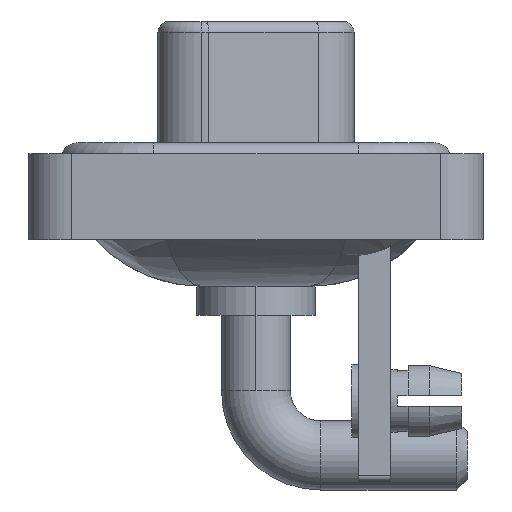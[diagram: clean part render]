
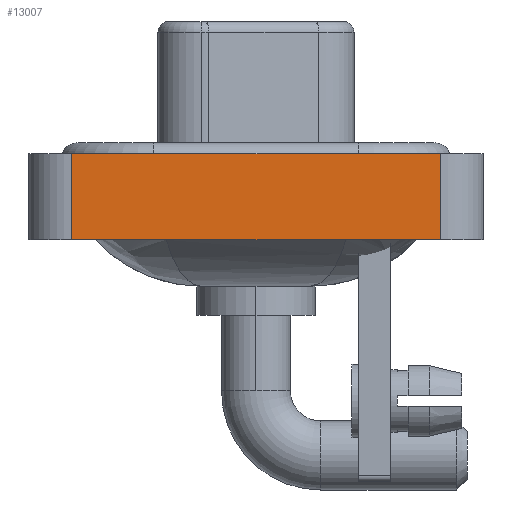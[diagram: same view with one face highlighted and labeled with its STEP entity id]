
A CAD part, left-side view. The second image highlights one B-rep face of the part: STEP entity #13007.
In plain terms, the highlighted planar face has unit normal (-1, 0, 0).
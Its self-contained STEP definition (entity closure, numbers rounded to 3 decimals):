
#25 = CARTESIAN_POINT ( 'NONE',  ( -7.35, -8.55, -3.6 ) ) ;
#1005 = AXIS2_PLACEMENT_3D ( 'NONE', #25, #5117, #6363 ) ;
#1102 = VERTEX_POINT ( 'NONE', #7436 ) ;
#1129 = CARTESIAN_POINT ( 'NONE',  ( -7.35, -8.55, -3.6 ) ) ;
#1330 = DIRECTION ( 'NONE',  ( 0., -1., 0. ) ) ;
#1501 = CARTESIAN_POINT ( 'NONE',  ( -7.35, -8.55, -3.6 ) ) ;
#2076 = VERTEX_POINT ( 'NONE', #9223 ) ;
#2586 = LINE ( 'NONE', #7348, #10680 ) ;
#2973 = ORIENTED_EDGE ( 'NONE', *, *, #6162, .T. ) ;
#3340 = PLANE ( 'NONE',  #1005 ) ;
#3378 = VECTOR ( 'NONE', #14199, 1000. ) ;
#4045 = ORIENTED_EDGE ( 'NONE', *, *, #5537, .F. ) ;
#4471 = VERTEX_POINT ( 'NONE', #8230 ) ;
#4541 = VECTOR ( 'NONE', #1330, 1000. ) ;
#5011 = ORIENTED_EDGE ( 'NONE', *, *, #11901, .T. ) ;
#5117 = DIRECTION ( 'NONE',  ( -1., 0., 0. ) ) ;
#5537 = EDGE_CURVE ( 'NONE', #1102, #2076, #2586, .T. ) ;
#6100 = DIRECTION ( 'NONE',  ( 0., 0., 1. ) ) ;
#6162 = EDGE_CURVE ( 'NONE', #13477, #4471, #7728, .T. ) ;
#6363 = DIRECTION ( 'NONE',  ( 0., 0., 1. ) ) ;
#6487 = EDGE_CURVE ( 'NONE', #2076, #4471, #10574, .T. ) ;
#7085 = ORIENTED_EDGE ( 'NONE', *, *, #6487, .F. ) ;
#7348 = CARTESIAN_POINT ( 'NONE',  ( -7.35, 8.55, -3.6 ) ) ;
#7436 = CARTESIAN_POINT ( 'NONE',  ( -7.35, 8.55, -3.6 ) ) ;
#7728 = LINE ( 'NONE', #1501, #13310 ) ;
#8230 = CARTESIAN_POINT ( 'NONE',  ( -7.35, -8.55, 0.4 ) ) ;
#9223 = CARTESIAN_POINT ( 'NONE',  ( -7.35, 8.55, 0.4 ) ) ;
#9279 = DIRECTION ( 'NONE',  ( 0., 0., 1. ) ) ;
#10574 = LINE ( 'NONE', #12130, #3378 ) ;
#10680 = VECTOR ( 'NONE', #6100, 1000. ) ;
#11901 = EDGE_CURVE ( 'NONE', #1102, #13477, #15318, .T. ) ;
#12130 = CARTESIAN_POINT ( 'NONE',  ( -7.35, -8.55, 0.4 ) ) ;
#13007 = ADVANCED_FACE ( 'NONE', ( #18965 ), #3340, .T. ) ;
#13310 = VECTOR ( 'NONE', #9279, 1000. ) ;
#13477 = VERTEX_POINT ( 'NONE', #14212 ) ;
#14199 = DIRECTION ( 'NONE',  ( 0., -1., 0. ) ) ;
#14212 = CARTESIAN_POINT ( 'NONE',  ( -7.35, -8.55, -3.6 ) ) ;
#15318 = LINE ( 'NONE', #1129, #4541 ) ;
#15506 = EDGE_LOOP ( 'NONE', ( #2973, #7085, #4045, #5011 ) ) ;
#18965 = FACE_OUTER_BOUND ( 'NONE', #15506, .T. ) ;
